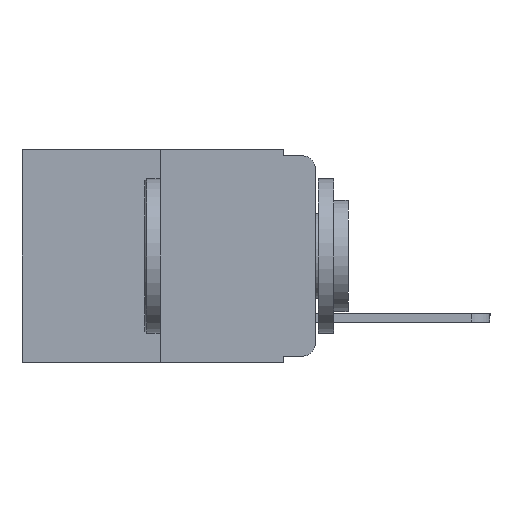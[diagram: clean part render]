
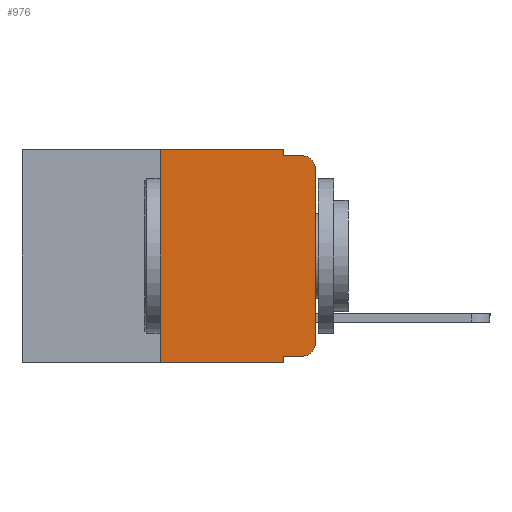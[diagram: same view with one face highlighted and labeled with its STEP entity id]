
A CAD part, left-side view. The second image highlights one B-rep face of the part: STEP entity #976.
In plain terms, the highlighted planar face has unit normal (-1, 0, 0).
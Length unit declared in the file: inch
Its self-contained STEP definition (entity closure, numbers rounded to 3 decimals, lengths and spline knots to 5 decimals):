
#125 = ORIENTED_EDGE ( 'NONE', *, *, #5328, .F. ) ;
#233 = LINE ( 'NONE', #7496, #632 ) ;
#367 = CARTESIAN_POINT ( 'NONE',  ( 0., 0.051, -0.01 ) ) ;
#412 = LINE ( 'NONE', #6752, #7978 ) ;
#430 = CARTESIAN_POINT ( 'NONE',  ( 0., 0.051, 0. ) ) ;
#632 = VECTOR ( 'NONE', #7468, 39.37008 ) ;
#792 = VERTEX_POINT ( 'NONE', #2758 ) ;
#976 = ADVANCED_FACE ( 'NONE', ( #8619 ), #7604, .F. ) ;
#1309 = DIRECTION ( 'NONE',  ( 0., 0., -1. ) ) ;
#1316 = DIRECTION ( 'NONE',  ( -1., 0., 0. ) ) ;
#1349 = CARTESIAN_POINT ( 'NONE',  ( 0., 0.02, -0.313 ) ) ;
#1368 = CARTESIAN_POINT ( 'NONE',  ( 0., 0.051, -0.333 ) ) ;
#1683 = ORIENTED_EDGE ( 'NONE', *, *, #4993, .F. ) ;
#1726 = DIRECTION ( 'NONE',  ( 0., -1., 0. ) ) ;
#1803 = DIRECTION ( 'NONE',  ( 0., -1., 0. ) ) ;
#1897 = VECTOR ( 'NONE', #6772, 39.37008 ) ;
#1955 = VERTEX_POINT ( 'NONE', #4672 ) ;
#2219 = CARTESIAN_POINT ( 'NONE',  ( 0., 0., 0. ) ) ;
#2506 = LINE ( 'NONE', #5116, #7506 ) ;
#2758 = CARTESIAN_POINT ( 'NONE',  ( 0., 0., -0.03 ) ) ;
#2808 = ORIENTED_EDGE ( 'NONE', *, *, #6018, .T. ) ;
#2898 = DIRECTION ( 'NONE',  ( 0., -1., 0. ) ) ;
#2993 = AXIS2_PLACEMENT_3D ( 'NONE', #1349, #1316, #1309 ) ;
#3310 = DIRECTION ( 'NONE',  ( 1., 0., 0. ) ) ;
#3387 = LINE ( 'NONE', #2219, #8583 ) ;
#3407 = VERTEX_POINT ( 'NONE', #9234 ) ;
#3497 = EDGE_CURVE ( 'NONE', #4653, #7144, #6482, .T. ) ;
#3800 = ORIENTED_EDGE ( 'NONE', *, *, #10867, .F. ) ;
#3834 = VERTEX_POINT ( 'NONE', #11969 ) ;
#3939 = VECTOR ( 'NONE', #4271, 39.37008 ) ;
#3992 = ORIENTED_EDGE ( 'NONE', *, *, #6499, .T. ) ;
#4271 = DIRECTION ( 'NONE',  ( 0., 0., -1. ) ) ;
#4366 = ORIENTED_EDGE ( 'NONE', *, *, #3497, .F. ) ;
#4372 = ORIENTED_EDGE ( 'NONE', *, *, #7972, .T. ) ;
#4544 = LINE ( 'NONE', #6447, #1897 ) ;
#4553 = ORIENTED_EDGE ( 'NONE', *, *, #8119, .T. ) ;
#4653 = VERTEX_POINT ( 'NONE', #367 ) ;
#4672 = CARTESIAN_POINT ( 'NONE',  ( 0., 0.051, 0. ) ) ;
#4716 = CARTESIAN_POINT ( 'NONE',  ( 0., 0., -0.313 ) ) ;
#4891 = EDGE_CURVE ( 'NONE', #1955, #4653, #233, .T. ) ;
#4937 = ORIENTED_EDGE ( 'NONE', *, *, #4891, .F. ) ;
#4993 = EDGE_CURVE ( 'NONE', #3834, #3407, #4544, .T. ) ;
#5116 = CARTESIAN_POINT ( 'NONE',  ( 0., 0.473, -0.343 ) ) ;
#5328 = EDGE_CURVE ( 'NONE', #6504, #11463, #6591, .T. ) ;
#5437 = DIRECTION ( 'NONE',  ( -1., 0., 0. ) ) ;
#5580 = CARTESIAN_POINT ( 'NONE',  ( 0., 0.051, -0.343 ) ) ;
#5672 = EDGE_LOOP ( 'NONE', ( #4372, #4553, #4366, #4937, #3800, #1683, #2808, #125, #11987, #3992 ) ) ;
#5759 = EDGE_CURVE ( 'NONE', #6504, #9509, #8232, .T. ) ;
#5970 = CARTESIAN_POINT ( 'NONE',  ( 0., 0.473, 0. ) ) ;
#6018 = EDGE_CURVE ( 'NONE', #3834, #11463, #2506, .T. ) ;
#6447 = CARTESIAN_POINT ( 'NONE',  ( 0., 0.25, 0. ) ) ;
#6482 = LINE ( 'NONE', #8530, #8682 ) ;
#6499 = EDGE_CURVE ( 'NONE', #9509, #10865, #9983, .T. ) ;
#6504 = VERTEX_POINT ( 'NONE', #1368 ) ;
#6591 = LINE ( 'NONE', #430, #3939 ) ;
#6654 = CARTESIAN_POINT ( 'NONE',  ( 0., 0.02, -0.333 ) ) ;
#6752 = CARTESIAN_POINT ( 'NONE',  ( 0., 0.473, 0. ) ) ;
#6772 = DIRECTION ( 'NONE',  ( 0., 0., 1. ) ) ;
#7030 = AXIS2_PLACEMENT_3D ( 'NONE', #5970, #3310, #12289 ) ;
#7144 = VERTEX_POINT ( 'NONE', #11635 ) ;
#7468 = DIRECTION ( 'NONE',  ( 0., 0., -1. ) ) ;
#7496 = CARTESIAN_POINT ( 'NONE',  ( 0., 0.051, 0. ) ) ;
#7506 = VECTOR ( 'NONE', #1803, 39.37008 ) ;
#7604 = PLANE ( 'NONE',  #7030 ) ;
#7972 = EDGE_CURVE ( 'NONE', #10865, #792, #3387, .T. ) ;
#7974 = AXIS2_PLACEMENT_3D ( 'NONE', #10962, #5437, #11760 ) ;
#7978 = VECTOR ( 'NONE', #1726, 39.37008 ) ;
#8116 = CARTESIAN_POINT ( 'NONE',  ( 0., 0.051, -0.333 ) ) ;
#8119 = EDGE_CURVE ( 'NONE', #792, #7144, #11517, .T. ) ;
#8134 = DIRECTION ( 'NONE',  ( 0., -1., 0. ) ) ;
#8232 = LINE ( 'NONE', #8116, #10288 ) ;
#8530 = CARTESIAN_POINT ( 'NONE',  ( 0., 0.051, -0.01 ) ) ;
#8583 = VECTOR ( 'NONE', #9034, 39.37008 ) ;
#8619 = FACE_OUTER_BOUND ( 'NONE', #5672, .T. ) ;
#8682 = VECTOR ( 'NONE', #2898, 39.37008 ) ;
#9034 = DIRECTION ( 'NONE',  ( 0., 0., 1. ) ) ;
#9234 = CARTESIAN_POINT ( 'NONE',  ( 0., 0.25, 0. ) ) ;
#9509 = VERTEX_POINT ( 'NONE', #6654 ) ;
#9983 = CIRCLE ( 'NONE', #2993, 0.02 ) ;
#10288 = VECTOR ( 'NONE', #8134, 39.37008 ) ;
#10865 = VERTEX_POINT ( 'NONE', #4716 ) ;
#10867 = EDGE_CURVE ( 'NONE', #3407, #1955, #412, .T. ) ;
#10962 = CARTESIAN_POINT ( 'NONE',  ( 0., 0.02, -0.03 ) ) ;
#11463 = VERTEX_POINT ( 'NONE', #5580 ) ;
#11517 = CIRCLE ( 'NONE', #7974, 0.02 ) ;
#11635 = CARTESIAN_POINT ( 'NONE',  ( 0., 0.02, -0.01 ) ) ;
#11760 = DIRECTION ( 'NONE',  ( 0., 0., -1. ) ) ;
#11969 = CARTESIAN_POINT ( 'NONE',  ( 0., 0.25, -0.343 ) ) ;
#11987 = ORIENTED_EDGE ( 'NONE', *, *, #5759, .T. ) ;
#12289 = DIRECTION ( 'NONE',  ( 0., 0., -1. ) ) ;
